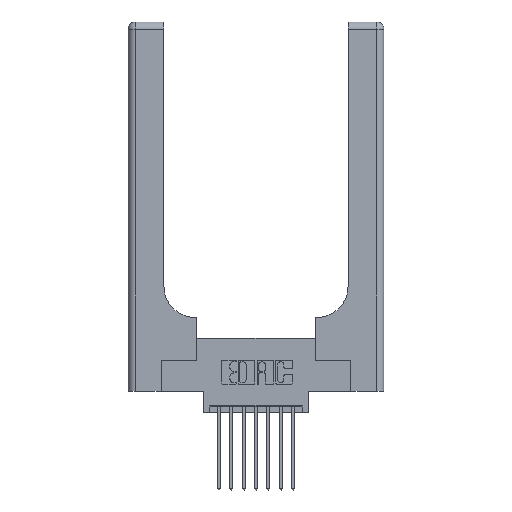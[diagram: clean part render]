
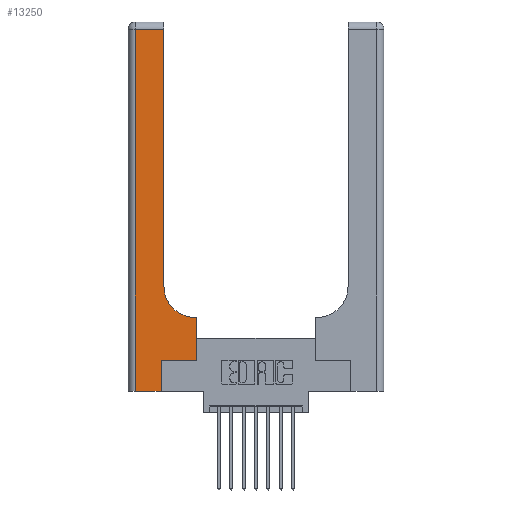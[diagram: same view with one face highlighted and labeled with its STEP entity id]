
A CAD part, top view. The second image highlights one B-rep face of the part: STEP entity #13250.
In plain terms, the highlighted planar face has unit normal (0, 0, 1).
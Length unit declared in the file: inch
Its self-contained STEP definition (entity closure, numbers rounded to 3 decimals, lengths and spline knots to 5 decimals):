
#58 = VECTOR ( 'NONE', #8474, 39.37008 ) ;
#123 = ORIENTED_EDGE ( 'NONE', *, *, #1287, .T. ) ;
#170 = EDGE_CURVE ( 'NONE', #7002, #12021, #9368, .T. ) ;
#252 = AXIS2_PLACEMENT_3D ( 'NONE', #13002, #9426, #2248 ) ;
#253 = VECTOR ( 'NONE', #11390, 39.37008 ) ;
#272 = LINE ( 'NONE', #13264, #9481 ) ;
#845 = ORIENTED_EDGE ( 'NONE', *, *, #5840, .T. ) ;
#1042 = PLANE ( 'NONE',  #252 ) ;
#1287 = EDGE_CURVE ( 'NONE', #12163, #12389, #2772, .T. ) ;
#1751 = VERTEX_POINT ( 'NONE', #8948 ) ;
#1948 = DIRECTION ( 'NONE',  ( 1., 0., 0. ) ) ;
#2036 = VECTOR ( 'NONE', #4406, 39.37008 ) ;
#2180 = CARTESIAN_POINT ( 'NONE',  ( 0.06, 2.94, 0.37 ) ) ;
#2248 = DIRECTION ( 'NONE',  ( -1., 0., 0. ) ) ;
#2500 = CARTESIAN_POINT ( 'NONE',  ( 0.06, 3., 0.37 ) ) ;
#2772 = LINE ( 'NONE', #13988, #10820 ) ;
#2785 = DIRECTION ( 'NONE',  ( 0., 0., -1. ) ) ;
#2865 = VECTOR ( 'NONE', #10205, 39.37008 ) ;
#2872 = CARTESIAN_POINT ( 'NONE',  ( 0.269, 0.25, 0.37 ) ) ;
#2885 = VERTEX_POINT ( 'NONE', #2180 ) ;
#3125 = CARTESIAN_POINT ( 'NONE',  ( 0., 0., 0.37 ) ) ;
#3176 = VERTEX_POINT ( 'NONE', #8668 ) ;
#3289 = LINE ( 'NONE', #2500, #58 ) ;
#3418 = LINE ( 'NONE', #9317, #10158 ) ;
#3872 = ORIENTED_EDGE ( 'NONE', *, *, #11606, .T. ) ;
#4406 = DIRECTION ( 'NONE',  ( 1., 0., 0. ) ) ;
#4425 = EDGE_CURVE ( 'NONE', #12021, #5987, #9603, .T. ) ;
#4633 = EDGE_CURVE ( 'NONE', #1751, #7002, #3418, .T. ) ;
#5816 = AXIS2_PLACEMENT_3D ( 'NONE', #14922, #2785, #13354 ) ;
#5840 = EDGE_CURVE ( 'NONE', #3176, #12163, #9772, .T. ) ;
#5987 = VERTEX_POINT ( 'NONE', #10544 ) ;
#6688 = LINE ( 'NONE', #8970, #253 ) ;
#7002 = VERTEX_POINT ( 'NONE', #11410 ) ;
#7121 = EDGE_CURVE ( 'NONE', #12389, #12180, #8790, .T. ) ;
#7883 = ORIENTED_EDGE ( 'NONE', *, *, #4633, .T. ) ;
#8161 = CARTESIAN_POINT ( 'NONE',  ( 0.269, 0., 0.37 ) ) ;
#8349 = ORIENTED_EDGE ( 'NONE', *, *, #170, .T. ) ;
#8474 = DIRECTION ( 'NONE',  ( 0., -1., 0. ) ) ;
#8510 = ORIENTED_EDGE ( 'NONE', *, *, #4425, .T. ) ;
#8668 = CARTESIAN_POINT ( 'NONE',  ( 0.06, 0., 0.37 ) ) ;
#8790 = LINE ( 'NONE', #12776, #2036 ) ;
#8843 = ORIENTED_EDGE ( 'NONE', *, *, #12309, .T. ) ;
#8948 = CARTESIAN_POINT ( 'NONE',  ( 0.5585, 0.6, 0.37 ) ) ;
#8952 = EDGE_LOOP ( 'NONE', ( #8510, #3872, #8843, #845, #123, #9646, #10555, #7883, #8349 ) ) ;
#8970 = CARTESIAN_POINT ( 'NONE',  ( 0.5585, 0.25, 0.37 ) ) ;
#8998 = CARTESIAN_POINT ( 'NONE',  ( 0.2915, 3., 0.37 ) ) ;
#9317 = CARTESIAN_POINT ( 'NONE',  ( 0.2915, 0.6, 0.37 ) ) ;
#9368 = CIRCLE ( 'NONE', #5816, 0.25 ) ;
#9426 = DIRECTION ( 'NONE',  ( 0., 0., -1. ) ) ;
#9481 = VECTOR ( 'NONE', #14477, 39.37008 ) ;
#9603 = LINE ( 'NONE', #8998, #2865 ) ;
#9646 = ORIENTED_EDGE ( 'NONE', *, *, #7121, .T. ) ;
#9772 = LINE ( 'NONE', #3125, #12584 ) ;
#10158 = VECTOR ( 'NONE', #15345, 39.37008 ) ;
#10205 = DIRECTION ( 'NONE',  ( 0., 1., 0. ) ) ;
#10544 = CARTESIAN_POINT ( 'NONE',  ( 0.2915, 2.94, 0.37 ) ) ;
#10555 = ORIENTED_EDGE ( 'NONE', *, *, #11297, .T. ) ;
#10820 = VECTOR ( 'NONE', #14100, 39.37008 ) ;
#11297 = EDGE_CURVE ( 'NONE', #12180, #1751, #6688, .T. ) ;
#11390 = DIRECTION ( 'NONE',  ( 0., 1., 0. ) ) ;
#11410 = CARTESIAN_POINT ( 'NONE',  ( 0.5415, 0.6, 0.37 ) ) ;
#11505 = FACE_OUTER_BOUND ( 'NONE', #8952, .T. ) ;
#11606 = EDGE_CURVE ( 'NONE', #5987, #2885, #272, .T. ) ;
#12021 = VERTEX_POINT ( 'NONE', #12680 ) ;
#12163 = VERTEX_POINT ( 'NONE', #8161 ) ;
#12180 = VERTEX_POINT ( 'NONE', #12985 ) ;
#12309 = EDGE_CURVE ( 'NONE', #2885, #3176, #3289, .T. ) ;
#12389 = VERTEX_POINT ( 'NONE', #2872 ) ;
#12584 = VECTOR ( 'NONE', #1948, 39.37008 ) ;
#12680 = CARTESIAN_POINT ( 'NONE',  ( 0.2915, 0.85, 0.37 ) ) ;
#12776 = CARTESIAN_POINT ( 'NONE',  ( 0.269, 0.25, 0.37 ) ) ;
#12985 = CARTESIAN_POINT ( 'NONE',  ( 0.5585, 0.25, 0.37 ) ) ;
#13002 = CARTESIAN_POINT ( 'NONE',  ( 0., 3., 0.37 ) ) ;
#13250 = ADVANCED_FACE ( 'NONE', ( #11505 ), #1042, .F. ) ;
#13264 = CARTESIAN_POINT ( 'NONE',  ( 0., 2.94, 0.37 ) ) ;
#13354 = DIRECTION ( 'NONE',  ( 1., 0., 0. ) ) ;
#13988 = CARTESIAN_POINT ( 'NONE',  ( 0.269, 0., 0.37 ) ) ;
#14100 = DIRECTION ( 'NONE',  ( 0., 1., 0. ) ) ;
#14477 = DIRECTION ( 'NONE',  ( -1., 0., 0. ) ) ;
#14922 = CARTESIAN_POINT ( 'NONE',  ( 0.5415, 0.85, 0.37 ) ) ;
#15345 = DIRECTION ( 'NONE',  ( -1., 0., 0. ) ) ;
